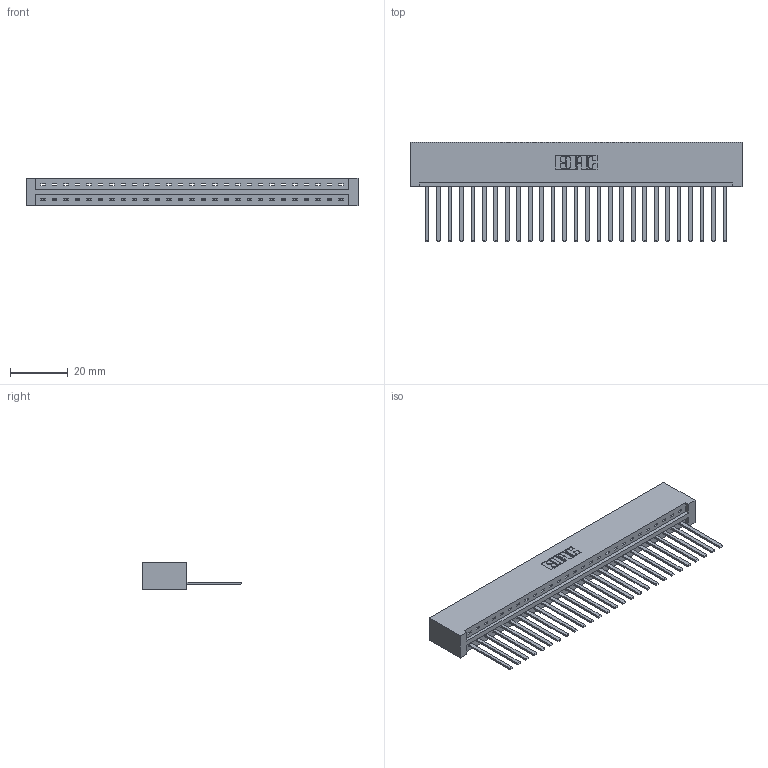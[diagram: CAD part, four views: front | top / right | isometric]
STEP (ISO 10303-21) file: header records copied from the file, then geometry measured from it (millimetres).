
FILE_DESCRIPTION (( 'STEP AP203' ), '1' );
FILE_NAME ('387-027-544-101.STEP', '2018-09-16T15:55:51', ( '' ), ( '' ), 'SwSTEP 2.0', 'SolidWorks 2016', '' );
FILE_SCHEMA (( 'CONFIG_CONTROL_DESIGN' ));
Length unit declared in the file: inch
Products named in the file (3): 337 Part_No Mounting Lugs; 345-292-001_345-293-144; 387-027-544-101
Assembly tree (28 placements, depth 2):
  387-027-544-101
    337 Part_No Mounting Lugs
    345-292-001_345-293-144  x27
Bounding box: 114.86 x 34.3 x 9.4 mm (x, y, z)
Volume: 12801.3 mm3; surface area: 14155.1 mm2
Topology: 28 solids, 28 shells, 1618 faces, 4877 edges, 3214 vertices
Faces by surface type: plane 1200, cylinder 418
Entity records: 21549 total; most frequent: CARTESIAN_POINT 3759, ORIENTED_EDGE 3722, DIRECTION 3183, EDGE_CURVE 1861, VECTOR 1745, LINE 1745, VERTEX_POINT 1238, AXIS2_PLACEMENT_3D 719
